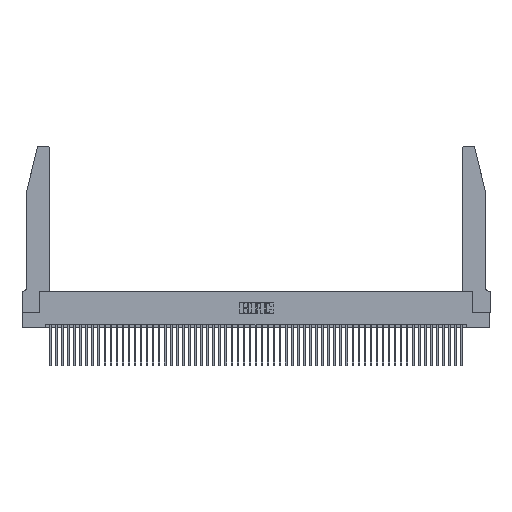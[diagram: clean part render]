
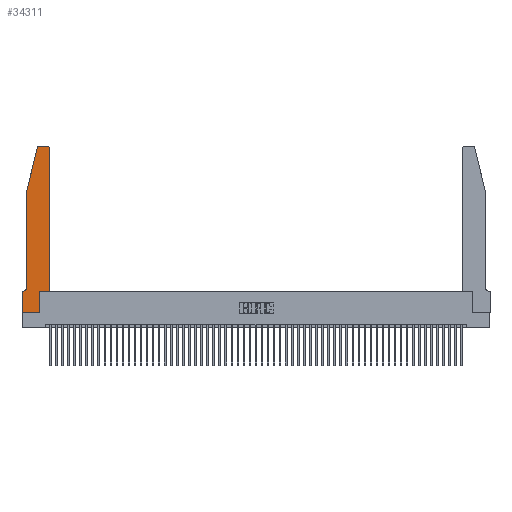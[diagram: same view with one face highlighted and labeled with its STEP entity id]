
A CAD part, top view. The second image highlights one B-rep face of the part: STEP entity #34311.
In plain terms, the highlighted planar face has unit normal (0, 0, 1).
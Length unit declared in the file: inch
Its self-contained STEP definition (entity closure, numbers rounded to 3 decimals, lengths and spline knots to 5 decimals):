
#662 = EDGE_CURVE ( 'NONE', #41449, #42134, #5033, .T. ) ;
#664 = EDGE_CURVE ( 'NONE', #17165, #41950, #38013, .T. ) ;
#728 = ORIENTED_EDGE ( 'NONE', *, *, #40270, .T. ) ;
#1514 = EDGE_CURVE ( 'NONE', #9124, #11559, #51676, .T. ) ;
#2339 = CARTESIAN_POINT ( 'NONE',  ( 0.4505, 0.35, 0.37 ) ) ;
#3228 = DIRECTION ( 'NONE',  ( 1., 0., 0. ) ) ;
#3533 = AXIS2_PLACEMENT_3D ( 'NONE', #47534, #22161, #51723 ) ;
#3707 = VECTOR ( 'NONE', #3228, 39.37008 ) ;
#3930 = LINE ( 'NONE', #44222, #15460 ) ;
#4117 = CARTESIAN_POINT ( 'NONE',  ( 0.25487, 2.72718, 0.37 ) ) ;
#5033 = LINE ( 'NONE', #16122, #26658 ) ;
#5191 = DIRECTION ( 'NONE',  ( -0.239, -0.971, 0. ) ) ;
#5284 = ORIENTED_EDGE ( 'NONE', *, *, #32311, .T. ) ;
#5506 = CIRCLE ( 'NONE', #42432, 0.03 ) ;
#5755 = DIRECTION ( 'NONE',  ( 0., 0., 1. ) ) ;
#6617 = ORIENTED_EDGE ( 'NONE', *, *, #16664, .T. ) ;
#7554 = VECTOR ( 'NONE', #9086, 39.37008 ) ;
#8483 = DIRECTION ( 'NONE',  ( 0., 0., 1. ) ) ;
#8816 = CARTESIAN_POINT ( 'NONE',  ( 0.0055, 0.35, 0.37 ) ) ;
#9086 = DIRECTION ( 'NONE',  ( 0., 1., 0. ) ) ;
#9124 = VERTEX_POINT ( 'NONE', #34761 ) ;
#9702 = CARTESIAN_POINT ( 'NONE',  ( 0., 0.35, 0.37 ) ) ;
#10038 = DIRECTION ( 'NONE',  ( -1., 0., 0. ) ) ;
#10950 = LINE ( 'NONE', #53573, #54884 ) ;
#11559 = VERTEX_POINT ( 'NONE', #38280 ) ;
#13016 = ORIENTED_EDGE ( 'NONE', *, *, #50154, .T. ) ;
#13557 = CIRCLE ( 'NONE', #21567, 0.03 ) ;
#14756 = ORIENTED_EDGE ( 'NONE', *, *, #664, .T. ) ;
#15208 = ORIENTED_EDGE ( 'NONE', *, *, #35823, .T. ) ;
#15460 = VECTOR ( 'NONE', #22893, 39.37008 ) ;
#16122 = CARTESIAN_POINT ( 'NONE',  ( 0.2605, 2.75, 0.37 ) ) ;
#16664 = EDGE_CURVE ( 'NONE', #31209, #41449, #13557, .T. ) ;
#17165 = VERTEX_POINT ( 'NONE', #47221 ) ;
#18785 = VERTEX_POINT ( 'NONE', #8816 ) ;
#19087 = VECTOR ( 'NONE', #10038, 39.37008 ) ;
#20513 = LINE ( 'NONE', #30519, #7554 ) ;
#20641 = DIRECTION ( 'NONE',  ( 0., 1., 0. ) ) ;
#20997 = EDGE_CURVE ( 'NONE', #41950, #31209, #20513, .T. ) ;
#21080 = VERTEX_POINT ( 'NONE', #30903 ) ;
#21567 = AXIS2_PLACEMENT_3D ( 'NONE', #31577, #5755, #35853 ) ;
#22161 = DIRECTION ( 'NONE',  ( 0., 0., -1. ) ) ;
#22286 = LINE ( 'NONE', #35293, #32264 ) ;
#22893 = DIRECTION ( 'NONE',  ( 0., -1., 0. ) ) ;
#24429 = VERTEX_POINT ( 'NONE', #4117 ) ;
#24519 = DIRECTION ( 'NONE',  ( 0., 0., 1. ) ) ;
#24738 = CARTESIAN_POINT ( 'NONE',  ( 0.2865, 0.35, 0.37 ) ) ;
#26658 = VECTOR ( 'NONE', #28874, 39.37008 ) ;
#27421 = EDGE_CURVE ( 'NONE', #30731, #21080, #10950, .T. ) ;
#28199 = CARTESIAN_POINT ( 'NONE',  ( 0.4205, 2.75, 0.37 ) ) ;
#28874 = DIRECTION ( 'NONE',  ( -1., 0., 0. ) ) ;
#29145 = VERTEX_POINT ( 'NONE', #9702 ) ;
#29553 = ORIENTED_EDGE ( 'NONE', *, *, #20997, .T. ) ;
#30184 = EDGE_CURVE ( 'NONE', #18785, #29145, #41715, .T. ) ;
#30519 = CARTESIAN_POINT ( 'NONE',  ( 0.4505, 0.35, 0.37 ) ) ;
#30731 = VERTEX_POINT ( 'NONE', #47465 ) ;
#30903 = CARTESIAN_POINT ( 'NONE',  ( 0.0755, 0.42, 0.37 ) ) ;
#31209 = VERTEX_POINT ( 'NONE', #42093 ) ;
#31449 = CARTESIAN_POINT ( 'NONE',  ( 0.0755, 0.35, 0.37 ) ) ;
#31577 = CARTESIAN_POINT ( 'NONE',  ( 0.4205, 2.72, 0.37 ) ) ;
#31852 = ORIENTED_EDGE ( 'NONE', *, *, #30184, .T. ) ;
#32238 = ORIENTED_EDGE ( 'NONE', *, *, #35666, .T. ) ;
#32264 = VECTOR ( 'NONE', #5191, 39.37008 ) ;
#32311 = EDGE_CURVE ( 'NONE', #11559, #17165, #35531, .T. ) ;
#32690 = CARTESIAN_POINT ( 'NONE',  ( 0., 0.35, 0.37 ) ) ;
#34128 = CARTESIAN_POINT ( 'NONE',  ( 0.284, 2.75, 0.37 ) ) ;
#34214 = VECTOR ( 'NONE', #20641, 39.37008 ) ;
#34252 = EDGE_LOOP ( 'NONE', ( #43467, #728, #13016, #49228, #32238, #31852, #15208, #44091, #5284, #14756, #29553, #6617 ) ) ;
#34264 = CARTESIAN_POINT ( 'NONE',  ( 0.284, 2.72, 0.37 ) ) ;
#34311 = ADVANCED_FACE ( 'NONE', ( #51826 ), #45646, .T. ) ;
#34761 = CARTESIAN_POINT ( 'NONE',  ( 0., 0., 0.37 ) ) ;
#35293 = CARTESIAN_POINT ( 'NONE',  ( 0.0755, 2., 0.37 ) ) ;
#35304 = DIRECTION ( 'NONE',  ( 1., 0., 0. ) ) ;
#35531 = LINE ( 'NONE', #24738, #34214 ) ;
#35666 = EDGE_CURVE ( 'NONE', #21080, #18785, #44824, .T. ) ;
#35823 = EDGE_CURVE ( 'NONE', #29145, #9124, #3930, .T. ) ;
#35853 = DIRECTION ( 'NONE',  ( 1., 0., 0. ) ) ;
#38013 = LINE ( 'NONE', #45901, #3707 ) ;
#38280 = CARTESIAN_POINT ( 'NONE',  ( 0.2865, 0., 0.37 ) ) ;
#38519 = DIRECTION ( 'NONE',  ( 1., 0., 0. ) ) ;
#40270 = EDGE_CURVE ( 'NONE', #42134, #24429, #5506, .T. ) ;
#40517 = VECTOR ( 'NONE', #35304, 39.37008 ) ;
#41449 = VERTEX_POINT ( 'NONE', #28199 ) ;
#41715 = LINE ( 'NONE', #31449, #19087 ) ;
#41950 = VERTEX_POINT ( 'NONE', #2339 ) ;
#42093 = CARTESIAN_POINT ( 'NONE',  ( 0.4505, 2.72, 0.37 ) ) ;
#42134 = VERTEX_POINT ( 'NONE', #34128 ) ;
#42432 = AXIS2_PLACEMENT_3D ( 'NONE', #34264, #8483, #38519 ) ;
#43467 = ORIENTED_EDGE ( 'NONE', *, *, #662, .T. ) ;
#44091 = ORIENTED_EDGE ( 'NONE', *, *, #1514, .T. ) ;
#44222 = CARTESIAN_POINT ( 'NONE',  ( 0., 0., 0.37 ) ) ;
#44824 = CIRCLE ( 'NONE', #3533, 0.07 ) ;
#45362 = DIRECTION ( 'NONE',  ( 0., -1., 0. ) ) ;
#45646 = PLANE ( 'NONE',  #51745 ) ;
#45901 = CARTESIAN_POINT ( 'NONE',  ( 0.4505, 0.35, 0.37 ) ) ;
#47221 = CARTESIAN_POINT ( 'NONE',  ( 0.2865, 0.35, 0.37 ) ) ;
#47465 = CARTESIAN_POINT ( 'NONE',  ( 0.0755, 2., 0.37 ) ) ;
#47534 = CARTESIAN_POINT ( 'NONE',  ( 0.0055, 0.42, 0.37 ) ) ;
#49228 = ORIENTED_EDGE ( 'NONE', *, *, #27421, .T. ) ;
#50154 = EDGE_CURVE ( 'NONE', #24429, #30731, #22286, .T. ) ;
#51676 = LINE ( 'NONE', #52041, #40517 ) ;
#51723 = DIRECTION ( 'NONE',  ( -1., 0., 0. ) ) ;
#51745 = AXIS2_PLACEMENT_3D ( 'NONE', #32690, #24519, #54051 ) ;
#51826 = FACE_OUTER_BOUND ( 'NONE', #34252, .T. ) ;
#52041 = CARTESIAN_POINT ( 'NONE',  ( 0., 0., 0.37 ) ) ;
#53573 = CARTESIAN_POINT ( 'NONE',  ( 0.0755, 2., 0.37 ) ) ;
#54051 = DIRECTION ( 'NONE',  ( 1., 0., 0. ) ) ;
#54884 = VECTOR ( 'NONE', #45362, 39.37008 ) ;
